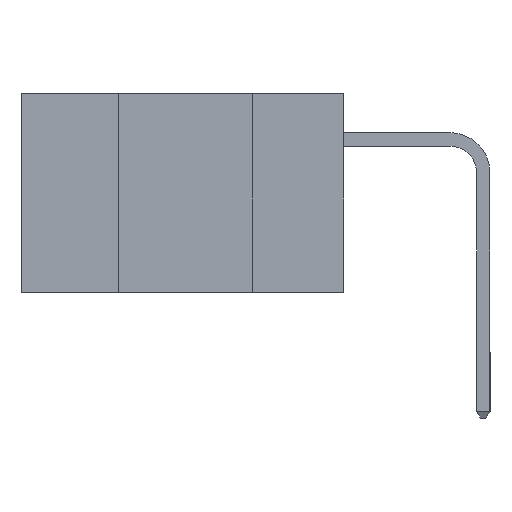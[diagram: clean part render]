
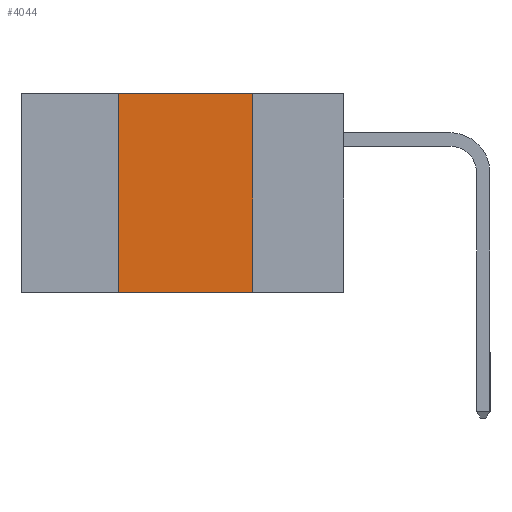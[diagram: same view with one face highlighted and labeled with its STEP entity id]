
A CAD part, left-side view. The second image highlights one B-rep face of the part: STEP entity #4044.
In plain terms, the highlighted planar face has unit normal (-1, 0, 0).
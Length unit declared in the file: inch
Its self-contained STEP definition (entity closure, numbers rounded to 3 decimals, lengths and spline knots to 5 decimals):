
#20 = LINE ( 'NONE', #2977, #13159 ) ;
#108 = VECTOR ( 'NONE', #6081, 39.37008 ) ;
#573 = DIRECTION ( 'NONE',  ( 1., 0., 0. ) ) ;
#642 = ORIENTED_EDGE ( 'NONE', *, *, #13392, .T. ) ;
#822 = EDGE_LOOP ( 'NONE', ( #6160, #1253, #3747, #642 ) ) ;
#1069 = LINE ( 'NONE', #5375, #15679 ) ;
#1253 = ORIENTED_EDGE ( 'NONE', *, *, #5416, .F. ) ;
#2528 = AXIS2_PLACEMENT_3D ( 'NONE', #3113, #573, #15214 ) ;
#2977 = CARTESIAN_POINT ( 'NONE',  ( 0., 0.6, -0.37 ) ) ;
#3113 = CARTESIAN_POINT ( 'NONE',  ( 0., 0.6, 0. ) ) ;
#3747 = ORIENTED_EDGE ( 'NONE', *, *, #16010, .F. ) ;
#3897 = VECTOR ( 'NONE', #11916, 39.37008 ) ;
#4044 = ADVANCED_FACE ( 'NONE', ( #16252 ), #16396, .F. ) ;
#5375 = CARTESIAN_POINT ( 'NONE',  ( 0., 0.17, 0. ) ) ;
#5416 = EDGE_CURVE ( 'NONE', #14570, #16767, #7159, .T. ) ;
#6057 = VERTEX_POINT ( 'NONE', #17263 ) ;
#6081 = DIRECTION ( 'NONE',  ( 0., -1., 0. ) ) ;
#6160 = ORIENTED_EDGE ( 'NONE', *, *, #13167, .F. ) ;
#6949 = CARTESIAN_POINT ( 'NONE',  ( 0., 0.42, -0.37 ) ) ;
#6970 = DIRECTION ( 'NONE',  ( 0., -1., 0. ) ) ;
#7159 = LINE ( 'NONE', #12835, #108 ) ;
#7660 = CARTESIAN_POINT ( 'NONE',  ( 0., 0.42, 0. ) ) ;
#7862 = LINE ( 'NONE', #14501, #3897 ) ;
#7973 = VERTEX_POINT ( 'NONE', #6949 ) ;
#11916 = DIRECTION ( 'NONE',  ( 0., 0., 1. ) ) ;
#12835 = CARTESIAN_POINT ( 'NONE',  ( 0., 0.6, 0. ) ) ;
#13159 = VECTOR ( 'NONE', #6970, 39.37008 ) ;
#13167 = EDGE_CURVE ( 'NONE', #16767, #6057, #1069, .T. ) ;
#13392 = EDGE_CURVE ( 'NONE', #7973, #6057, #20, .T. ) ;
#14501 = CARTESIAN_POINT ( 'NONE',  ( 0., 0.42, 0. ) ) ;
#14570 = VERTEX_POINT ( 'NONE', #7660 ) ;
#14684 = DIRECTION ( 'NONE',  ( 0., 0., -1. ) ) ;
#15214 = DIRECTION ( 'NONE',  ( 0., 0., -1. ) ) ;
#15679 = VECTOR ( 'NONE', #14684, 39.37008 ) ;
#15777 = CARTESIAN_POINT ( 'NONE',  ( 0., 0.17, 0. ) ) ;
#16010 = EDGE_CURVE ( 'NONE', #7973, #14570, #7862, .T. ) ;
#16252 = FACE_OUTER_BOUND ( 'NONE', #822, .T. ) ;
#16396 = PLANE ( 'NONE',  #2528 ) ;
#16767 = VERTEX_POINT ( 'NONE', #15777 ) ;
#17263 = CARTESIAN_POINT ( 'NONE',  ( 0., 0.17, -0.37 ) ) ;
